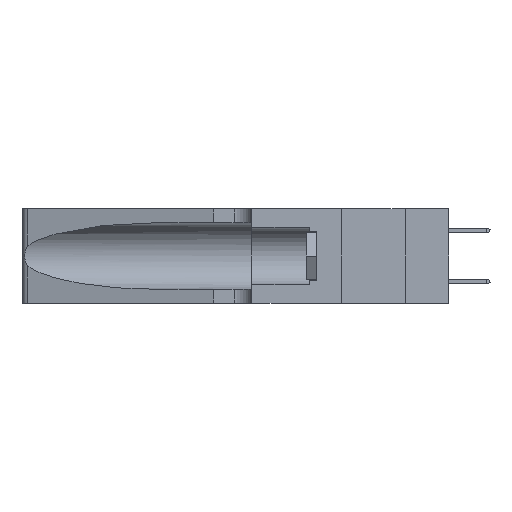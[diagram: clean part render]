
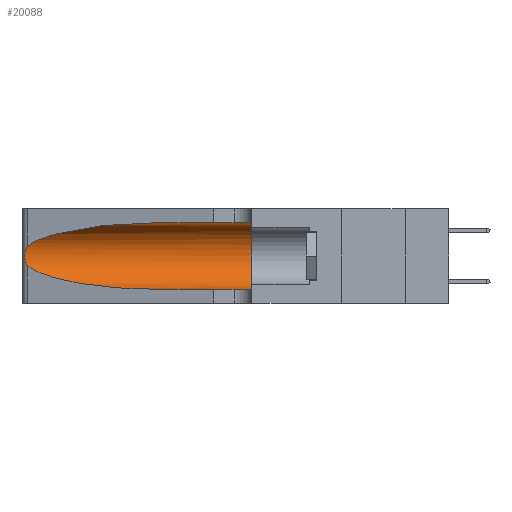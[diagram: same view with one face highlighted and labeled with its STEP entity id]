
A CAD part, left-side view. The second image highlights one B-rep face of the part: STEP entity #20088.
In plain terms, the highlighted cylindrical face has radius 3.308 mm (diameter 6.617 mm), a partial arc.
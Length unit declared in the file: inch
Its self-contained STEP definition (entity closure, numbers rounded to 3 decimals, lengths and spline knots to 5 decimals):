
#57 = CARTESIAN_POINT ( 'NONE',  ( 0.25854, 1.2359, 0.20912 ) ) ;
#222 = CARTESIAN_POINT ( 'NONE',  ( 0.1305, 0.35, 0.185 ) ) ;
#564 = CARTESIAN_POINT ( 'NONE',  ( 0.1305, 0.72297, 0.05475 ) ) ;
#1397 = AXIS2_PLACEMENT_3D ( 'NONE', #222, #8251, #22734 ) ;
#1720 = VECTOR ( 'NONE', #5851, 39.37008 ) ;
#1776 = CARTESIAN_POINT ( 'NONE',  ( 0.2373, 1.15595, 0.08982 ) ) ;
#2570 = VERTEX_POINT ( 'NONE', #22559 ) ;
#2808 = ORIENTED_EDGE ( 'NONE', *, *, #13177, .F. ) ;
#3883 = CARTESIAN_POINT ( 'NONE',  ( 0.26075, 1.23896, 0.178 ) ) ;
#3884 = ORIENTED_EDGE ( 'NONE', *, *, #8261, .T. ) ;
#3914 = CYLINDRICAL_SURFACE ( 'NONE', #24339, 0.13025 ) ;
#4636 = CARTESIAN_POINT ( 'NONE',  ( 0.25487, 1.22718, 0.14631 ) ) ;
#4756 = VERTEX_POINT ( 'NONE', #564 ) ;
#5851 = DIRECTION ( 'NONE',  ( 0., -1., 0. ) ) ;
#5981 = EDGE_LOOP ( 'NONE', ( #8116, #3884, #19397, #6814, #2808, #18715 ) ) ;
#6156 = CARTESIAN_POINT ( 'NONE',  ( 0.25555, 1.22993, 0.14849 ) ) ;
#6324 = CARTESIAN_POINT ( 'NONE',  ( 0.26075, 1.23896, 0.19203 ) ) ;
#6814 = ORIENTED_EDGE ( 'NONE', *, *, #20316, .T. ) ;
#6901 =( BOUNDED_CURVE ( )  B_SPLINE_CURVE ( 3, ( #18869, #12825, #8331, #20959 ),
 .UNSPECIFIED., .F., .F. ) 
 B_SPLINE_CURVE_WITH_KNOTS ( ( 4, 4 ),
 ( 1.5708, 2.84003 ),
 .UNSPECIFIED. ) 
 CURVE ( )  GEOMETRIC_REPRESENTATION_ITEM ( )  RATIONAL_B_SPLINE_CURVE ( ( 1., 0.87, 0.87, 1. ) ) 
 REPRESENTATION_ITEM ( '' )  );
#7409 = DIRECTION ( 'NONE',  ( 0., -1., 0. ) ) ;
#8116 = ORIENTED_EDGE ( 'NONE', *, *, #23990, .T. ) ;
#8250 = CARTESIAN_POINT ( 'NONE',  ( 0.25856, 1.23593, 0.16098 ) ) ;
#8251 = DIRECTION ( 'NONE',  ( 0., 1., 0. ) ) ;
#8261 = EDGE_CURVE ( 'NONE', #19042, #9781, #26536, .T. ) ;
#8331 = CARTESIAN_POINT ( 'NONE',  ( 0.2373, 1.15595, 0.28018 ) ) ;
#9493 = DIRECTION ( 'NONE',  ( 0., 0., -1. ) ) ;
#9781 = VERTEX_POINT ( 'NONE', #4636 ) ;
#10057 = CARTESIAN_POINT ( 'NONE',  ( 0.25487, 1.22718, 0.14631 ) ) ;
#10326 = CARTESIAN_POINT ( 'NONE',  ( 0.25787, 1.23484, 0.2124 ) ) ;
#11462 = CARTESIAN_POINT ( 'NONE',  ( 0.1305, 1.61858, 0.185 ) ) ;
#11926 = CARTESIAN_POINT ( 'NONE',  ( 0.1305, 1.61858, 0.31525 ) ) ;
#12039 = FACE_OUTER_BOUND ( 'NONE', #5981, .T. ) ;
#12405 = CARTESIAN_POINT ( 'NONE',  ( 0.26018, 1.23835, 0.19895 ) ) ;
#12463 = LINE ( 'NONE', #11926, #1720 ) ;
#12825 = CARTESIAN_POINT ( 'NONE',  ( 0.18966, 0.96281, 0.31525 ) ) ;
#13177 = EDGE_CURVE ( 'NONE', #19112, #16332, #20997, .T. ) ;
#13336 = LINE ( 'NONE', #24343, #23037 ) ;
#14022 = CARTESIAN_POINT ( 'NONE',  ( 0.18966, 0.96281, 0.05475 ) ) ;
#14203 = CARTESIAN_POINT ( 'NONE',  ( 0.25487, 1.22718, 0.14631 ) ) ;
#16288 = CARTESIAN_POINT ( 'NONE',  ( 0.25639, 1.23184, 0.21858 ) ) ;
#16332 = VERTEX_POINT ( 'NONE', #17099 ) ;
#16780 = EDGE_CURVE ( 'NONE', #9781, #4756, #19657, .T. ) ;
#17099 = CARTESIAN_POINT ( 'NONE',  ( 0.1305, 0.35, 0.05475 ) ) ;
#18353 = CARTESIAN_POINT ( 'NONE',  ( 0.25487, 1.22718, 0.22369 ) ) ;
#18715 = ORIENTED_EDGE ( 'NONE', *, *, #19514, .F. ) ;
#18869 = CARTESIAN_POINT ( 'NONE',  ( 0.1305, 0.72297, 0.31525 ) ) ;
#18873 = CARTESIAN_POINT ( 'NONE',  ( 0.25487, 1.22718, 0.22369 ) ) ;
#19042 = VERTEX_POINT ( 'NONE', #18873 ) ;
#19112 = VERTEX_POINT ( 'NONE', #19224 ) ;
#19224 = CARTESIAN_POINT ( 'NONE',  ( 0.1305, 0.35, 0.31525 ) ) ;
#19397 = ORIENTED_EDGE ( 'NONE', *, *, #16780, .T. ) ;
#19514 = EDGE_CURVE ( 'NONE', #2570, #19112, #12463, .T. ) ;
#19657 =( BOUNDED_CURVE ( )  B_SPLINE_CURVE ( 3, ( #14203, #1776, #14022, #24363 ),
 .UNSPECIFIED., .F., .T. ) 
 B_SPLINE_CURVE_WITH_KNOTS ( ( 4, 4 ),
 ( 3.44316, 4.71239 ),
 .UNSPECIFIED. ) 
 CURVE ( )  GEOMETRIC_REPRESENTATION_ITEM ( )  RATIONAL_B_SPLINE_CURVE ( ( 1., 0.87, 0.87, 1. ) ) 
 REPRESENTATION_ITEM ( '' )  );
#20088 = ADVANCED_FACE ( 'NONE', ( #12039 ), #3914, .F. ) ;
#20316 = EDGE_CURVE ( 'NONE', #4756, #16332, #13336, .T. ) ;
#20438 = CARTESIAN_POINT ( 'NONE',  ( 0.25789, 1.23486, 0.15765 ) ) ;
#20623 = CARTESIAN_POINT ( 'NONE',  ( 0.25639, 1.23186, 0.15144 ) ) ;
#20710 = CARTESIAN_POINT ( 'NONE',  ( 0.26017, 1.23833, 0.17102 ) ) ;
#20959 = CARTESIAN_POINT ( 'NONE',  ( 0.25487, 1.22718, 0.22369 ) ) ;
#20997 = CIRCLE ( 'NONE', #1397, 0.13025 ) ;
#22559 = CARTESIAN_POINT ( 'NONE',  ( 0.1305, 0.72297, 0.31525 ) ) ;
#22732 = CARTESIAN_POINT ( 'NONE',  ( 0.25555, 1.22994, 0.2215 ) ) ;
#22734 = DIRECTION ( 'NONE',  ( 0., 0., 1. ) ) ;
#23037 = VECTOR ( 'NONE', #26555, 39.37008 ) ;
#23990 = EDGE_CURVE ( 'NONE', #2570, #19042, #6901, .T. ) ;
#24339 = AXIS2_PLACEMENT_3D ( 'NONE', #11462, #7409, #9493 ) ;
#24343 = CARTESIAN_POINT ( 'NONE',  ( 0.1305, 1.61858, 0.05475 ) ) ;
#24363 = CARTESIAN_POINT ( 'NONE',  ( 0.1305, 0.72297, 0.05475 ) ) ;
#26536 = B_SPLINE_CURVE_WITH_KNOTS ( 'NONE', 3,
 ( #18353, #22732, #16288, #10326, #57, #12405, #6324, #3883, #20710, #8250, #20438, #20623, #6156, #10057 ),
 .UNSPECIFIED., .F., .F.,
 ( 4, 2, 2, 2, 2, 2, 4 ),
 ( 0., 0.00027, 0.00053, 0.00107, 0.0016, 0.00187, 0.00214 ),
 .UNSPECIFIED. ) ;
#26555 = DIRECTION ( 'NONE',  ( 0., -1., 0. ) ) ;
